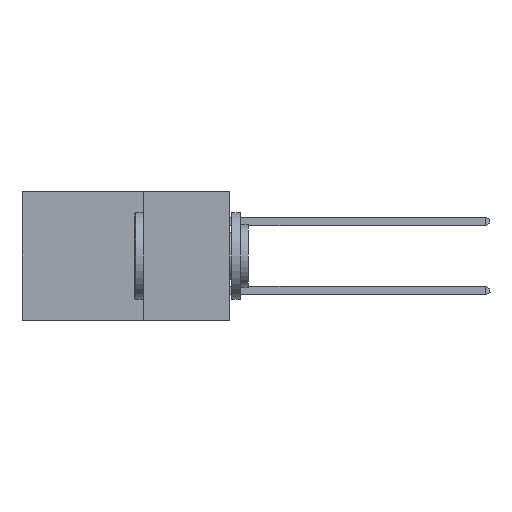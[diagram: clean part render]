
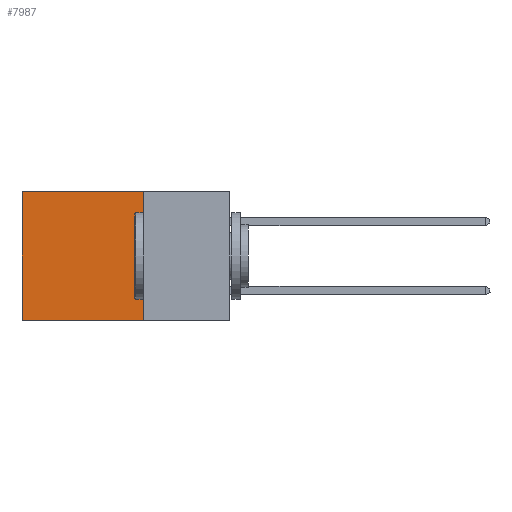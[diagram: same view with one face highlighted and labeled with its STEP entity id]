
A CAD part, left-side view. The second image highlights one B-rep face of the part: STEP entity #7987.
In plain terms, the highlighted planar face has unit normal (-1, 0, 0).
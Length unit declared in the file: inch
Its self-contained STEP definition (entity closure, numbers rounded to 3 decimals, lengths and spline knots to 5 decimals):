
#656 = CARTESIAN_POINT ( 'NONE',  ( 0.298, 0.25, -0.37 ) ) ;
#993 = VERTEX_POINT ( 'NONE', #12723 ) ;
#2291 = EDGE_CURVE ( 'NONE', #12747, #10046, #3868, .T. ) ;
#3457 = DIRECTION ( 'NONE',  ( 0., 0., -1. ) ) ;
#3645 = CARTESIAN_POINT ( 'NONE',  ( 0.298, 0.6, 0. ) ) ;
#3689 = DIRECTION ( 'NONE',  ( 0., 0., -1. ) ) ;
#3868 = LINE ( 'NONE', #656, #8882 ) ;
#4077 = VECTOR ( 'NONE', #5666, 39.37008 ) ;
#4686 = VECTOR ( 'NONE', #3689, 39.37008 ) ;
#4823 = DIRECTION ( 'NONE',  ( 0., 1., 0. ) ) ;
#4879 = VECTOR ( 'NONE', #9466, 39.37008 ) ;
#4885 = ORIENTED_EDGE ( 'NONE', *, *, #7715, .F. ) ;
#5666 = DIRECTION ( 'NONE',  ( 0., 1., 0. ) ) ;
#5879 = FACE_OUTER_BOUND ( 'NONE', #11828, .T. ) ;
#6142 = EDGE_CURVE ( 'NONE', #8939, #993, #12407, .T. ) ;
#6149 = AXIS2_PLACEMENT_3D ( 'NONE', #13155, #12979, #3457 ) ;
#6206 = CARTESIAN_POINT ( 'NONE',  ( 0.298, 0.25, -0.37 ) ) ;
#6789 = PLANE ( 'NONE',  #6149 ) ;
#7715 = EDGE_CURVE ( 'NONE', #8939, #12747, #12545, .T. ) ;
#7987 = ADVANCED_FACE ( 'NONE', ( #5879 ), #6789, .F. ) ;
#8868 = CARTESIAN_POINT ( 'NONE',  ( 0.298, 0.6, -0.37 ) ) ;
#8882 = VECTOR ( 'NONE', #4823, 39.37008 ) ;
#8884 = LINE ( 'NONE', #3645, #4686 ) ;
#8939 = VERTEX_POINT ( 'NONE', #10631 ) ;
#9360 = ORIENTED_EDGE ( 'NONE', *, *, #6142, .T. ) ;
#9466 = DIRECTION ( 'NONE',  ( 0., 0., -1. ) ) ;
#9638 = ORIENTED_EDGE ( 'NONE', *, *, #2291, .F. ) ;
#10046 = VERTEX_POINT ( 'NONE', #8868 ) ;
#10631 = CARTESIAN_POINT ( 'NONE',  ( 0.298, 0.25, 0. ) ) ;
#11542 = CARTESIAN_POINT ( 'NONE',  ( 0.298, 0.25, 0. ) ) ;
#11712 = ORIENTED_EDGE ( 'NONE', *, *, #13134, .T. ) ;
#11828 = EDGE_LOOP ( 'NONE', ( #11712, #9638, #4885, #9360 ) ) ;
#12407 = LINE ( 'NONE', #13050, #4077 ) ;
#12545 = LINE ( 'NONE', #11542, #4879 ) ;
#12723 = CARTESIAN_POINT ( 'NONE',  ( 0.298, 0.6, 0. ) ) ;
#12747 = VERTEX_POINT ( 'NONE', #6206 ) ;
#12979 = DIRECTION ( 'NONE',  ( 1., 0., 0. ) ) ;
#13050 = CARTESIAN_POINT ( 'NONE',  ( 0.298, 0.25, 0. ) ) ;
#13134 = EDGE_CURVE ( 'NONE', #993, #10046, #8884, .T. ) ;
#13155 = CARTESIAN_POINT ( 'NONE',  ( 0.298, 0.25, 0. ) ) ;
